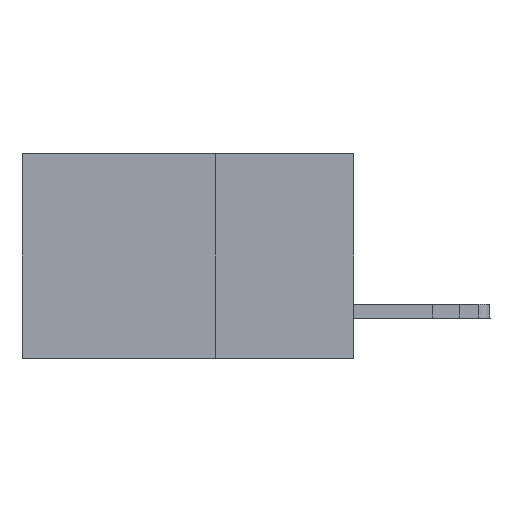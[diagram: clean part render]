
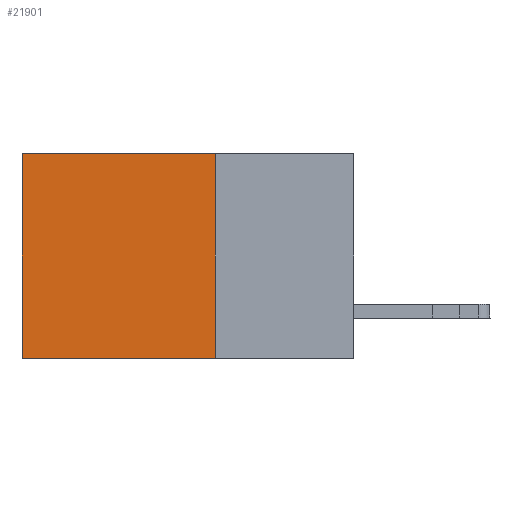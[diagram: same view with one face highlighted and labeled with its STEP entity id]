
A CAD part, left-side view. The second image highlights one B-rep face of the part: STEP entity #21901.
In plain terms, the highlighted planar face has unit normal (-1, 0, 0).
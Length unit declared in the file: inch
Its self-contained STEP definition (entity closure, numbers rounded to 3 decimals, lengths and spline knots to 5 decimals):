
#981 = EDGE_CURVE ( 'NONE', #12425, #6365, #20989, .T. ) ;
#1546 = AXIS2_PLACEMENT_3D ( 'NONE', #21946, #5462, #3533 ) ;
#1975 = ORIENTED_EDGE ( 'NONE', *, *, #16379, .F. ) ;
#2065 = DIRECTION ( 'NONE',  ( 0., 0., -1. ) ) ;
#3240 = DIRECTION ( 'NONE',  ( 0., 1., 0. ) ) ;
#3533 = DIRECTION ( 'NONE',  ( 0., 0., -1. ) ) ;
#5462 = DIRECTION ( 'NONE',  ( 1., 0., 0. ) ) ;
#6210 = CARTESIAN_POINT ( 'NONE',  ( 0.2875, 0.6, 0. ) ) ;
#6365 = VERTEX_POINT ( 'NONE', #12739 ) ;
#6588 = CARTESIAN_POINT ( 'NONE',  ( 0.2875, 0.25, -0.37 ) ) ;
#7186 = ORIENTED_EDGE ( 'NONE', *, *, #981, .T. ) ;
#8055 = VERTEX_POINT ( 'NONE', #14341 ) ;
#8741 = CARTESIAN_POINT ( 'NONE',  ( 0.2875, 0.25, 0. ) ) ;
#9365 = FACE_OUTER_BOUND ( 'NONE', #19179, .T. ) ;
#11207 = EDGE_CURVE ( 'NONE', #8055, #12425, #19860, .T. ) ;
#11246 = ORIENTED_EDGE ( 'NONE', *, *, #11207, .T. ) ;
#11597 = VERTEX_POINT ( 'NONE', #22547 ) ;
#12425 = VERTEX_POINT ( 'NONE', #15126 ) ;
#12464 = LINE ( 'NONE', #19906, #16823 ) ;
#12739 = CARTESIAN_POINT ( 'NONE',  ( 0.2875, 0.6, -0.37 ) ) ;
#13506 = DIRECTION ( 'NONE',  ( 0., 0., -1. ) ) ;
#14341 = CARTESIAN_POINT ( 'NONE',  ( 0.2875, 0.25, 0. ) ) ;
#15126 = CARTESIAN_POINT ( 'NONE',  ( 0.2875, 0.6, 0. ) ) ;
#16249 = ORIENTED_EDGE ( 'NONE', *, *, #16396, .F. ) ;
#16379 = EDGE_CURVE ( 'NONE', #11597, #6365, #21707, .T. ) ;
#16396 = EDGE_CURVE ( 'NONE', #8055, #11597, #12464, .T. ) ;
#16823 = VECTOR ( 'NONE', #13506, 39.37008 ) ;
#18795 = VECTOR ( 'NONE', #23320, 39.37008 ) ;
#19179 = EDGE_LOOP ( 'NONE', ( #7186, #1975, #16249, #11246 ) ) ;
#19268 = VECTOR ( 'NONE', #3240, 39.37008 ) ;
#19860 = LINE ( 'NONE', #8741, #19268 ) ;
#19906 = CARTESIAN_POINT ( 'NONE',  ( 0.2875, 0.25, 0. ) ) ;
#20126 = PLANE ( 'NONE',  #1546 ) ;
#20457 = VECTOR ( 'NONE', #2065, 39.37008 ) ;
#20989 = LINE ( 'NONE', #6210, #20457 ) ;
#21707 = LINE ( 'NONE', #6588, #18795 ) ;
#21901 = ADVANCED_FACE ( 'NONE', ( #9365 ), #20126, .F. ) ;
#21946 = CARTESIAN_POINT ( 'NONE',  ( 0.2875, 0.25, 0. ) ) ;
#22547 = CARTESIAN_POINT ( 'NONE',  ( 0.2875, 0.25, -0.37 ) ) ;
#23320 = DIRECTION ( 'NONE',  ( 0., 1., 0. ) ) ;
